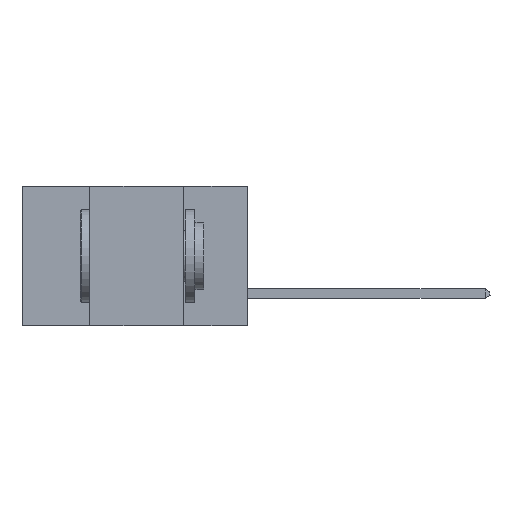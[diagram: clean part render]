
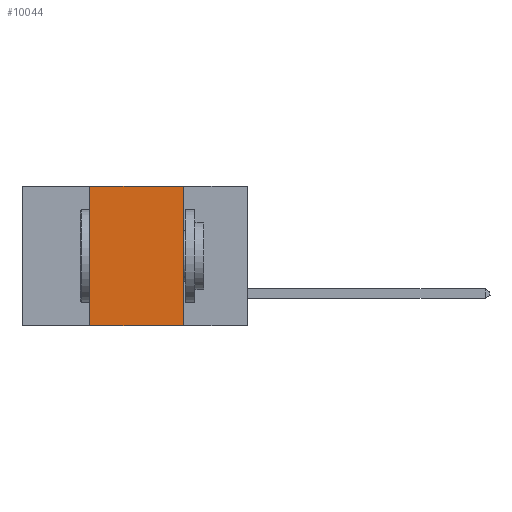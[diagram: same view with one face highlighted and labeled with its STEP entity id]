
A CAD part, left-side view. The second image highlights one B-rep face of the part: STEP entity #10044.
In plain terms, the highlighted planar face has unit normal (-1, 0, 0).
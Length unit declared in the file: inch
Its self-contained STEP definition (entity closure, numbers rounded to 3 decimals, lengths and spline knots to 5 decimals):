
#691 = VERTEX_POINT ( 'NONE', #10457 ) ;
#795 = ORIENTED_EDGE ( 'NONE', *, *, #11391, .F. ) ;
#1287 = VECTOR ( 'NONE', #4342, 39.37008 ) ;
#1331 = CARTESIAN_POINT ( 'NONE',  ( 0., 0.6, 0. ) ) ;
#1551 = CARTESIAN_POINT ( 'NONE',  ( 0., 0.6, 0. ) ) ;
#1573 = LINE ( 'NONE', #14646, #8847 ) ;
#1837 = FACE_OUTER_BOUND ( 'NONE', #10872, .T. ) ;
#2705 = CARTESIAN_POINT ( 'NONE',  ( 0., 0.17, 0. ) ) ;
#3226 = DIRECTION ( 'NONE',  ( 0., 0., -1. ) ) ;
#3410 = ORIENTED_EDGE ( 'NONE', *, *, #19934, .F. ) ;
#4342 = DIRECTION ( 'NONE',  ( 0., 0., -1. ) ) ;
#5818 = VERTEX_POINT ( 'NONE', #12366 ) ;
#6117 = EDGE_CURVE ( 'NONE', #14440, #8795, #16600, .T. ) ;
#6286 = DIRECTION ( 'NONE',  ( 0., 0., 1. ) ) ;
#7540 = CARTESIAN_POINT ( 'NONE',  ( 0., 0.42, -0.37 ) ) ;
#8795 = VERTEX_POINT ( 'NONE', #21242 ) ;
#8847 = VECTOR ( 'NONE', #6286, 39.37008 ) ;
#9864 = PLANE ( 'NONE',  #14267 ) ;
#10044 = ADVANCED_FACE ( 'NONE', ( #1837 ), #9864, .F. ) ;
#10457 = CARTESIAN_POINT ( 'NONE',  ( 0., 0.42, 0. ) ) ;
#10872 = EDGE_LOOP ( 'NONE', ( #19646, #795, #3410, #12973 ) ) ;
#11391 = EDGE_CURVE ( 'NONE', #691, #5818, #16097, .T. ) ;
#11464 = DIRECTION ( 'NONE',  ( 1., 0., 0. ) ) ;
#12160 = VECTOR ( 'NONE', #14067, 39.37008 ) ;
#12366 = CARTESIAN_POINT ( 'NONE',  ( 0., 0.17, 0. ) ) ;
#12973 = ORIENTED_EDGE ( 'NONE', *, *, #6117, .T. ) ;
#13238 = VECTOR ( 'NONE', #17899, 39.37008 ) ;
#14067 = DIRECTION ( 'NONE',  ( 0., -1., 0. ) ) ;
#14267 = AXIS2_PLACEMENT_3D ( 'NONE', #1551, #11464, #3226 ) ;
#14440 = VERTEX_POINT ( 'NONE', #7540 ) ;
#14541 = LINE ( 'NONE', #2705, #1287 ) ;
#14646 = CARTESIAN_POINT ( 'NONE',  ( 0., 0.42, 0. ) ) ;
#15447 = CARTESIAN_POINT ( 'NONE',  ( 0., 0.6, -0.37 ) ) ;
#16097 = LINE ( 'NONE', #1331, #13238 ) ;
#16600 = LINE ( 'NONE', #15447, #12160 ) ;
#17899 = DIRECTION ( 'NONE',  ( 0., -1., 0. ) ) ;
#19646 = ORIENTED_EDGE ( 'NONE', *, *, #20393, .F. ) ;
#19934 = EDGE_CURVE ( 'NONE', #14440, #691, #1573, .T. ) ;
#20393 = EDGE_CURVE ( 'NONE', #5818, #8795, #14541, .T. ) ;
#21242 = CARTESIAN_POINT ( 'NONE',  ( 0., 0.17, -0.37 ) ) ;
